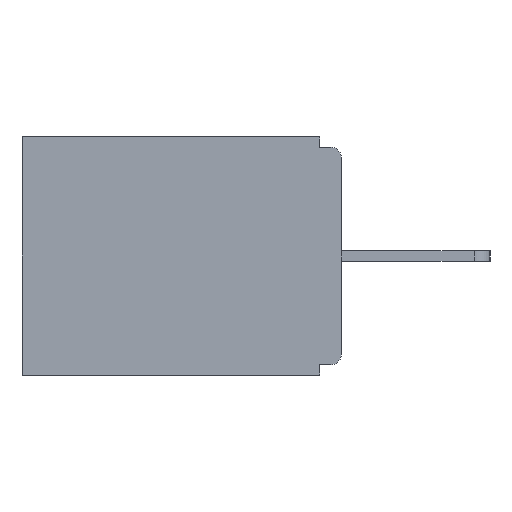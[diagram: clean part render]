
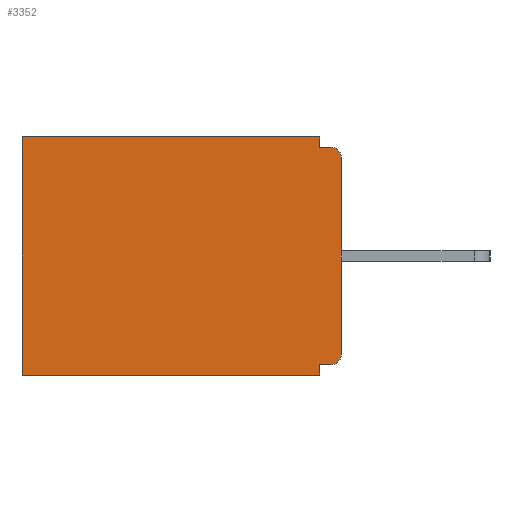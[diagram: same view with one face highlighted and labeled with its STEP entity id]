
A CAD part, left-side view. The second image highlights one B-rep face of the part: STEP entity #3352.
In plain terms, the highlighted planar face has unit normal (-1, 0, 0).
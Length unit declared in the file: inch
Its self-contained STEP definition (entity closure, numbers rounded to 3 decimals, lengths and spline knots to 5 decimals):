
#197 = VERTEX_POINT ( 'NONE', #532 ) ;
#327 = VERTEX_POINT ( 'NONE', #11167 ) ;
#377 = EDGE_CURVE ( 'NONE', #327, #12065, #9200, .T. ) ;
#532 = CARTESIAN_POINT ( 'NONE',  ( 0.298, 0.46, 0. ) ) ;
#618 = ORIENTED_EDGE ( 'NONE', *, *, #12089, .T. ) ;
#671 = DIRECTION ( 'NONE',  ( -1., 0., 0. ) ) ;
#937 = EDGE_CURVE ( 'NONE', #8779, #2691, #5852, .T. ) ;
#964 = EDGE_CURVE ( 'NONE', #4499, #11495, #1132, .T. ) ;
#1132 = LINE ( 'NONE', #9514, #9513 ) ;
#1135 = CARTESIAN_POINT ( 'NONE',  ( 0.298, 0.015, -0.328 ) ) ;
#1460 = ORIENTED_EDGE ( 'NONE', *, *, #5032, .F. ) ;
#1859 = ORIENTED_EDGE ( 'NONE', *, *, #9786, .F. ) ;
#1944 = CARTESIAN_POINT ( 'NONE',  ( 0.298, 0., 0. ) ) ;
#1983 = DIRECTION ( 'NONE',  ( 0., 1., 0. ) ) ;
#2529 = CARTESIAN_POINT ( 'NONE',  ( 0.298, 0.015, -0.313 ) ) ;
#2691 = VERTEX_POINT ( 'NONE', #5738 ) ;
#2832 = DIRECTION ( 'NONE',  ( 0., -1., 0. ) ) ;
#2842 = PLANE ( 'NONE',  #14225 ) ;
#3352 = ADVANCED_FACE ( 'NONE', ( #14412 ), #2842, .F. ) ;
#3623 = DIRECTION ( 'NONE',  ( 0., 1., 0. ) ) ;
#3879 = CARTESIAN_POINT ( 'NONE',  ( 0.298, 0.46, 0. ) ) ;
#4346 = CARTESIAN_POINT ( 'NONE',  ( 0.298, 0.46, -0.343 ) ) ;
#4442 = CIRCLE ( 'NONE', #7545, 0.015 ) ;
#4451 = CARTESIAN_POINT ( 'NONE',  ( 0.298, 0.031, -0.343 ) ) ;
#4467 = VECTOR ( 'NONE', #8246, 39.37008 ) ;
#4499 = VERTEX_POINT ( 'NONE', #6649 ) ;
#4752 = DIRECTION ( 'NONE',  ( -1., 0., 0. ) ) ;
#4834 = ORIENTED_EDGE ( 'NONE', *, *, #11547, .T. ) ;
#5032 = EDGE_CURVE ( 'NONE', #12794, #12735, #14500, .T. ) ;
#5124 = CARTESIAN_POINT ( 'NONE',  ( 0.298, 0., 0. ) ) ;
#5738 = CARTESIAN_POINT ( 'NONE',  ( 0.298, 0.031, -0.328 ) ) ;
#5760 = CARTESIAN_POINT ( 'NONE',  ( 0.298, 0., 0. ) ) ;
#5852 = LINE ( 'NONE', #10260, #12867 ) ;
#5931 = DIRECTION ( 'NONE',  ( 0., 0., -1. ) ) ;
#5953 = LINE ( 'NONE', #3879, #6089 ) ;
#6089 = VECTOR ( 'NONE', #8414, 39.37008 ) ;
#6215 = DIRECTION ( 'NONE',  ( 0., 0., -1. ) ) ;
#6426 = EDGE_CURVE ( 'NONE', #8779, #12065, #13339, .T. ) ;
#6439 = DIRECTION ( 'NONE',  ( 0., 1., 0. ) ) ;
#6649 = CARTESIAN_POINT ( 'NONE',  ( 0.298, 0.031, -0.343 ) ) ;
#7179 = ORIENTED_EDGE ( 'NONE', *, *, #377, .F. ) ;
#7372 = DIRECTION ( 'NONE',  ( 0., 0., -1. ) ) ;
#7541 = VECTOR ( 'NONE', #8795, 39.37008 ) ;
#7545 = AXIS2_PLACEMENT_3D ( 'NONE', #14159, #671, #6215 ) ;
#7549 = AXIS2_PLACEMENT_3D ( 'NONE', #2529, #4752, #5931 ) ;
#7700 = CARTESIAN_POINT ( 'NONE',  ( 0.298, 0.031, -0.015 ) ) ;
#8246 = DIRECTION ( 'NONE',  ( 0., 0., -1. ) ) ;
#8397 = LINE ( 'NONE', #9736, #12556 ) ;
#8414 = DIRECTION ( 'NONE',  ( 0., 0., -1. ) ) ;
#8513 = VECTOR ( 'NONE', #6439, 39.37008 ) ;
#8541 = VERTEX_POINT ( 'NONE', #8650 ) ;
#8575 = ORIENTED_EDGE ( 'NONE', *, *, #937, .F. ) ;
#8632 = DIRECTION ( 'NONE',  ( 1., 0., 0. ) ) ;
#8640 = ORIENTED_EDGE ( 'NONE', *, *, #964, .F. ) ;
#8650 = CARTESIAN_POINT ( 'NONE',  ( 0.298, 0.015, -0.015 ) ) ;
#8779 = VERTEX_POINT ( 'NONE', #1135 ) ;
#8795 = DIRECTION ( 'NONE',  ( 0., 0., -1. ) ) ;
#9200 = LINE ( 'NONE', #5760, #4467 ) ;
#9513 = VECTOR ( 'NONE', #3623, 39.37008 ) ;
#9514 = CARTESIAN_POINT ( 'NONE',  ( 0.298, 0., -0.343 ) ) ;
#9589 = DIRECTION ( 'NONE',  ( 0., 0., -1. ) ) ;
#9736 = CARTESIAN_POINT ( 'NONE',  ( 0.298, 0.031, -0.343 ) ) ;
#9786 = EDGE_CURVE ( 'NONE', #12735, #8541, #14262, .T. ) ;
#9842 = EDGE_LOOP ( 'NONE', ( #13833, #1859, #1460, #4834, #618, #8640, #14509, #8575, #12650, #7179 ) ) ;
#10260 = CARTESIAN_POINT ( 'NONE',  ( 0.298, 0., -0.328 ) ) ;
#11064 = CARTESIAN_POINT ( 'NONE',  ( 0.298, 0.031, 0. ) ) ;
#11167 = CARTESIAN_POINT ( 'NONE',  ( 0.298, 0., -0.03 ) ) ;
#11412 = EDGE_CURVE ( 'NONE', #327, #8541, #4442, .T. ) ;
#11495 = VERTEX_POINT ( 'NONE', #4346 ) ;
#11547 = EDGE_CURVE ( 'NONE', #12794, #197, #12147, .T. ) ;
#12065 = VERTEX_POINT ( 'NONE', #14118 ) ;
#12089 = EDGE_CURVE ( 'NONE', #197, #11495, #5953, .T. ) ;
#12147 = LINE ( 'NONE', #1944, #8513 ) ;
#12288 = VECTOR ( 'NONE', #2832, 39.37008 ) ;
#12556 = VECTOR ( 'NONE', #9589, 39.37008 ) ;
#12640 = EDGE_CURVE ( 'NONE', #2691, #4499, #8397, .T. ) ;
#12650 = ORIENTED_EDGE ( 'NONE', *, *, #6426, .T. ) ;
#12735 = VERTEX_POINT ( 'NONE', #7700 ) ;
#12794 = VERTEX_POINT ( 'NONE', #11064 ) ;
#12867 = VECTOR ( 'NONE', #1983, 39.37008 ) ;
#13135 = CARTESIAN_POINT ( 'NONE',  ( 0.298, 0., -0.015 ) ) ;
#13339 = CIRCLE ( 'NONE', #7549, 0.015 ) ;
#13833 = ORIENTED_EDGE ( 'NONE', *, *, #11412, .T. ) ;
#14118 = CARTESIAN_POINT ( 'NONE',  ( 0.298, 0., -0.313 ) ) ;
#14159 = CARTESIAN_POINT ( 'NONE',  ( 0.298, 0.015, -0.03 ) ) ;
#14225 = AXIS2_PLACEMENT_3D ( 'NONE', #5124, #8632, #7372 ) ;
#14262 = LINE ( 'NONE', #13135, #12288 ) ;
#14412 = FACE_OUTER_BOUND ( 'NONE', #9842, .T. ) ;
#14500 = LINE ( 'NONE', #4451, #7541 ) ;
#14509 = ORIENTED_EDGE ( 'NONE', *, *, #12640, .F. ) ;
